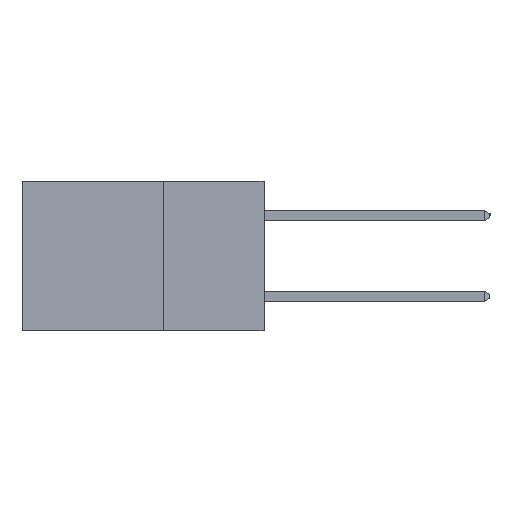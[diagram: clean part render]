
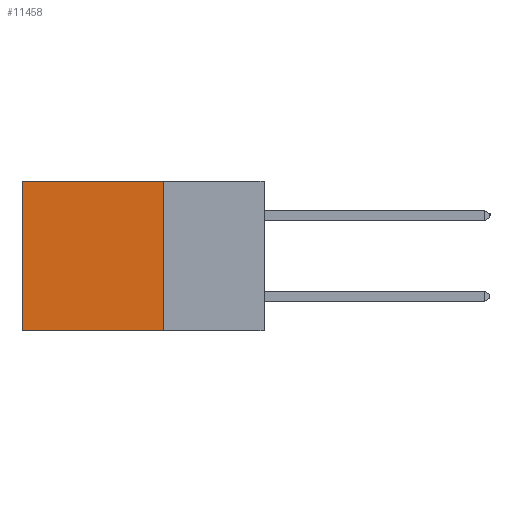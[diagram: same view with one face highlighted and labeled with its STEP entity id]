
A CAD part, left-side view. The second image highlights one B-rep face of the part: STEP entity #11458.
In plain terms, the highlighted planar face has unit normal (-1, 0, 0).
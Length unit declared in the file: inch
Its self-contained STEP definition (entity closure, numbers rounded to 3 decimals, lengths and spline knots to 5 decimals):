
#336 = DIRECTION ( 'NONE',  ( 1., 0., 0. ) ) ;
#818 = AXIS2_PLACEMENT_3D ( 'NONE', #11138, #336, #2108 ) ;
#839 = EDGE_CURVE ( 'NONE', #6732, #10922, #4359, .T. ) ;
#1020 = VECTOR ( 'NONE', #10466, 39.37008 ) ;
#1542 = CARTESIAN_POINT ( 'NONE',  ( 0.2615, 0.6, 0. ) ) ;
#2019 = VECTOR ( 'NONE', #7937, 39.37008 ) ;
#2108 = DIRECTION ( 'NONE',  ( 0., 0., -1. ) ) ;
#2503 = CARTESIAN_POINT ( 'NONE',  ( 0.2615, 0.25, -0.37 ) ) ;
#2609 = DIRECTION ( 'NONE',  ( 0., 0., -1. ) ) ;
#4359 = LINE ( 'NONE', #2503, #2019 ) ;
#4435 = CARTESIAN_POINT ( 'NONE',  ( 0.2615, 0.25, -0.37 ) ) ;
#4518 = EDGE_CURVE ( 'NONE', #7005, #10922, #11701, .T. ) ;
#4537 = ORIENTED_EDGE ( 'NONE', *, *, #4518, .T. ) ;
#5525 = FACE_OUTER_BOUND ( 'NONE', #10034, .T. ) ;
#6604 = EDGE_CURVE ( 'NONE', #11289, #6732, #9400, .T. ) ;
#6732 = VERTEX_POINT ( 'NONE', #4435 ) ;
#6828 = CARTESIAN_POINT ( 'NONE',  ( 0.2615, 0.25, -0.37 ) ) ;
#7005 = VERTEX_POINT ( 'NONE', #1542 ) ;
#7106 = EDGE_CURVE ( 'NONE', #11289, #7005, #7148, .T. ) ;
#7148 = LINE ( 'NONE', #9950, #10362 ) ;
#7937 = DIRECTION ( 'NONE',  ( 0., 1., 0. ) ) ;
#8152 = ORIENTED_EDGE ( 'NONE', *, *, #6604, .F. ) ;
#8268 = CARTESIAN_POINT ( 'NONE',  ( 0.2615, 0.6, -0.37 ) ) ;
#8520 = CARTESIAN_POINT ( 'NONE',  ( 0.2615, 0.25, 0. ) ) ;
#8949 = DIRECTION ( 'NONE',  ( 0., 1., 0. ) ) ;
#9400 = LINE ( 'NONE', #6828, #1020 ) ;
#9950 = CARTESIAN_POINT ( 'NONE',  ( 0.2615, 0.25, 0. ) ) ;
#10034 = EDGE_LOOP ( 'NONE', ( #4537, #11037, #8152, #10046 ) ) ;
#10046 = ORIENTED_EDGE ( 'NONE', *, *, #7106, .T. ) ;
#10061 = CARTESIAN_POINT ( 'NONE',  ( 0.2615, 0.6, -0.37 ) ) ;
#10105 = PLANE ( 'NONE',  #818 ) ;
#10362 = VECTOR ( 'NONE', #8949, 39.37008 ) ;
#10466 = DIRECTION ( 'NONE',  ( 0., 0., -1. ) ) ;
#10922 = VERTEX_POINT ( 'NONE', #8268 ) ;
#11037 = ORIENTED_EDGE ( 'NONE', *, *, #839, .F. ) ;
#11138 = CARTESIAN_POINT ( 'NONE',  ( 0.2615, 0.25, -0.37 ) ) ;
#11289 = VERTEX_POINT ( 'NONE', #8520 ) ;
#11458 = ADVANCED_FACE ( 'NONE', ( #5525 ), #10105, .F. ) ;
#11553 = VECTOR ( 'NONE', #2609, 39.37008 ) ;
#11701 = LINE ( 'NONE', #10061, #11553 ) ;
